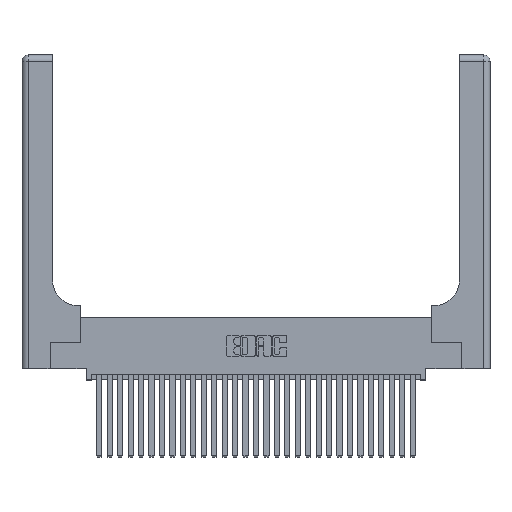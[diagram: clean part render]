
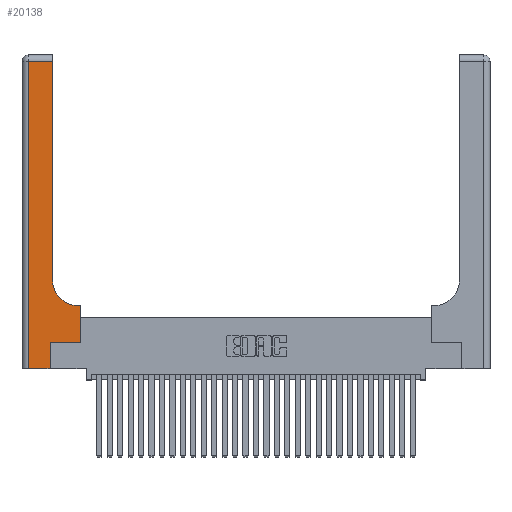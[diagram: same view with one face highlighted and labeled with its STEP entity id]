
A CAD part, top view. The second image highlights one B-rep face of the part: STEP entity #20138.
In plain terms, the highlighted planar face has unit normal (0, 0, 1).
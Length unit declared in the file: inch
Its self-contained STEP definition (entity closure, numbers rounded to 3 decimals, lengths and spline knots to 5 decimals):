
#1121 = ORIENTED_EDGE ( 'NONE', *, *, #27978, .T. ) ;
#1589 = LINE ( 'NONE', #2968, #15197 ) ;
#1853 = CARTESIAN_POINT ( 'NONE',  ( 0., 0., 0.37 ) ) ;
#2061 = VERTEX_POINT ( 'NONE', #7817 ) ;
#2171 = CARTESIAN_POINT ( 'NONE',  ( 0., 3., 0.37 ) ) ;
#2551 = VERTEX_POINT ( 'NONE', #11742 ) ;
#2643 = EDGE_CURVE ( 'NONE', #12378, #22591, #29873, .T. ) ;
#2780 = VECTOR ( 'NONE', #13723, 39.37008 ) ;
#2968 = CARTESIAN_POINT ( 'NONE',  ( 0.269, 0.25, 0.37 ) ) ;
#3253 = LINE ( 'NONE', #10157, #15270 ) ;
#3875 = VECTOR ( 'NONE', #28686, 39.37008 ) ;
#3921 = VECTOR ( 'NONE', #17476, 39.37008 ) ;
#4666 = DIRECTION ( 'NONE',  ( -1., 0., 0. ) ) ;
#5006 = ORIENTED_EDGE ( 'NONE', *, *, #8257, .T. ) ;
#5430 = DIRECTION ( 'NONE',  ( 1., 0., 0. ) ) ;
#5576 = CARTESIAN_POINT ( 'NONE',  ( 0., 2.94, 0.37 ) ) ;
#5856 = LINE ( 'NONE', #27559, #11482 ) ;
#7227 = AXIS2_PLACEMENT_3D ( 'NONE', #2171, #18975, #4666 ) ;
#7334 = VERTEX_POINT ( 'NONE', #8403 ) ;
#7746 = VECTOR ( 'NONE', #29669, 39.37008 ) ;
#7817 = CARTESIAN_POINT ( 'NONE',  ( 0.5415, 0.6, 0.37 ) ) ;
#8171 = EDGE_CURVE ( 'NONE', #23284, #2551, #5856, .T. ) ;
#8257 = EDGE_CURVE ( 'NONE', #2551, #2061, #9986, .T. ) ;
#8403 = CARTESIAN_POINT ( 'NONE',  ( 0.2915, 0.85, 0.37 ) ) ;
#8757 = DIRECTION ( 'NONE',  ( 0., 0., -1. ) ) ;
#9068 = VERTEX_POINT ( 'NONE', #16563 ) ;
#9179 = ORIENTED_EDGE ( 'NONE', *, *, #12437, .T. ) ;
#9986 = LINE ( 'NONE', #25492, #2780 ) ;
#10157 = CARTESIAN_POINT ( 'NONE',  ( 0.06, 3., 0.37 ) ) ;
#10616 = CARTESIAN_POINT ( 'NONE',  ( 0.269, 0.25, 0.37 ) ) ;
#11171 = VERTEX_POINT ( 'NONE', #25963 ) ;
#11482 = VECTOR ( 'NONE', #13408, 39.37008 ) ;
#11742 = CARTESIAN_POINT ( 'NONE',  ( 0.5585, 0.6, 0.37 ) ) ;
#11784 = VECTOR ( 'NONE', #13915, 39.37008 ) ;
#12154 = CARTESIAN_POINT ( 'NONE',  ( 0.269, 0., 0.37 ) ) ;
#12378 = VERTEX_POINT ( 'NONE', #20879 ) ;
#12437 = EDGE_CURVE ( 'NONE', #23723, #12378, #12539, .T. ) ;
#12539 = LINE ( 'NONE', #1853, #11784 ) ;
#12560 = DIRECTION ( 'NONE',  ( 0., -1., 0. ) ) ;
#13408 = DIRECTION ( 'NONE',  ( 0., 1., 0. ) ) ;
#13723 = DIRECTION ( 'NONE',  ( -1., 0., 0. ) ) ;
#13915 = DIRECTION ( 'NONE',  ( 1., 0., 0. ) ) ;
#14073 = LINE ( 'NONE', #24939, #7746 ) ;
#14719 = EDGE_CURVE ( 'NONE', #2061, #7334, #30896, .T. ) ;
#15197 = VECTOR ( 'NONE', #5430, 39.37008 ) ;
#15270 = VECTOR ( 'NONE', #12560, 39.37008 ) ;
#15495 = ORIENTED_EDGE ( 'NONE', *, *, #2643, .T. ) ;
#16563 = CARTESIAN_POINT ( 'NONE',  ( 0.06, 2.94, 0.37 ) ) ;
#16625 = LINE ( 'NONE', #5576, #3921 ) ;
#17476 = DIRECTION ( 'NONE',  ( -1., 0., 0. ) ) ;
#18975 = DIRECTION ( 'NONE',  ( 0., 0., -1. ) ) ;
#19897 = AXIS2_PLACEMENT_3D ( 'NONE', #22967, #8757, #25323 ) ;
#20138 = ADVANCED_FACE ( 'NONE', ( #29972 ), #28347, .F. ) ;
#20512 = EDGE_CURVE ( 'NONE', #7334, #11171, #14073, .T. ) ;
#20879 = CARTESIAN_POINT ( 'NONE',  ( 0.269, 0., 0.37 ) ) ;
#21104 = EDGE_CURVE ( 'NONE', #11171, #9068, #16625, .T. ) ;
#21818 = ORIENTED_EDGE ( 'NONE', *, *, #29770, .T. ) ;
#22591 = VERTEX_POINT ( 'NONE', #10616 ) ;
#22967 = CARTESIAN_POINT ( 'NONE',  ( 0.5415, 0.85, 0.37 ) ) ;
#23284 = VERTEX_POINT ( 'NONE', #24981 ) ;
#23723 = VERTEX_POINT ( 'NONE', #27024 ) ;
#24367 = ORIENTED_EDGE ( 'NONE', *, *, #20512, .T. ) ;
#24747 = ORIENTED_EDGE ( 'NONE', *, *, #14719, .T. ) ;
#24939 = CARTESIAN_POINT ( 'NONE',  ( 0.2915, 3., 0.37 ) ) ;
#24981 = CARTESIAN_POINT ( 'NONE',  ( 0.5585, 0.25, 0.37 ) ) ;
#25323 = DIRECTION ( 'NONE',  ( 1., 0., 0. ) ) ;
#25492 = CARTESIAN_POINT ( 'NONE',  ( 0.2915, 0.6, 0.37 ) ) ;
#25843 = ORIENTED_EDGE ( 'NONE', *, *, #21104, .T. ) ;
#25963 = CARTESIAN_POINT ( 'NONE',  ( 0.2915, 2.94, 0.37 ) ) ;
#26131 = EDGE_LOOP ( 'NONE', ( #24367, #25843, #1121, #9179, #15495, #21818, #29533, #5006, #24747 ) ) ;
#27024 = CARTESIAN_POINT ( 'NONE',  ( 0.06, 0., 0.37 ) ) ;
#27559 = CARTESIAN_POINT ( 'NONE',  ( 0.5585, 0.25, 0.37 ) ) ;
#27978 = EDGE_CURVE ( 'NONE', #9068, #23723, #3253, .T. ) ;
#28347 = PLANE ( 'NONE',  #7227 ) ;
#28686 = DIRECTION ( 'NONE',  ( 0., 1., 0. ) ) ;
#29533 = ORIENTED_EDGE ( 'NONE', *, *, #8171, .T. ) ;
#29669 = DIRECTION ( 'NONE',  ( 0., 1., 0. ) ) ;
#29770 = EDGE_CURVE ( 'NONE', #22591, #23284, #1589, .T. ) ;
#29873 = LINE ( 'NONE', #12154, #3875 ) ;
#29972 = FACE_OUTER_BOUND ( 'NONE', #26131, .T. ) ;
#30896 = CIRCLE ( 'NONE', #19897, 0.25 ) ;
